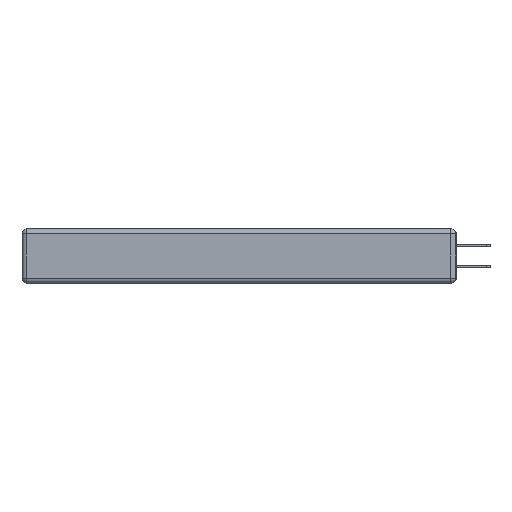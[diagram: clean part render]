
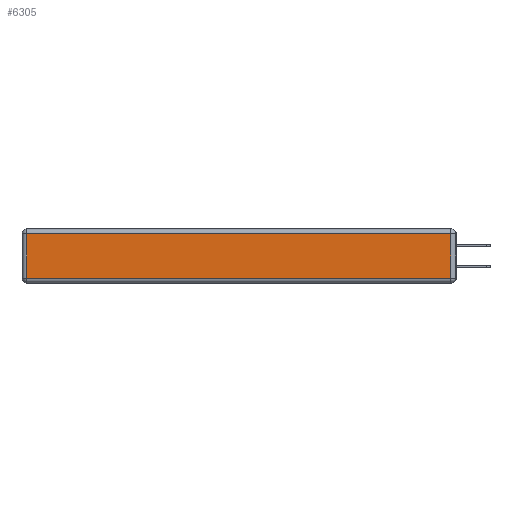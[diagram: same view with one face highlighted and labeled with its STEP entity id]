
A CAD part, left-side view. The second image highlights one B-rep face of the part: STEP entity #6305.
In plain terms, the highlighted planar face has unit normal (-1, 0, 0).
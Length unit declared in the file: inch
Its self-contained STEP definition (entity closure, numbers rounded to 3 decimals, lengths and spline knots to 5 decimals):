
#382 = LINE ( 'NONE', #2606, #5823 ) ;
#821 = ORIENTED_EDGE ( 'NONE', *, *, #4009, .T. ) ;
#872 = LINE ( 'NONE', #3025, #12431 ) ;
#1055 = EDGE_CURVE ( 'NONE', #5582, #9117, #6219, .T. ) ;
#1303 = VERTEX_POINT ( 'NONE', #5323 ) ;
#2340 = CARTESIAN_POINT ( 'NONE',  ( 0., 2.72, -0.313 ) ) ;
#2557 = DIRECTION ( 'NONE',  ( 0., 0., 1. ) ) ;
#2606 = CARTESIAN_POINT ( 'NONE',  ( 0., 0.03, -0.343 ) ) ;
#3025 = CARTESIAN_POINT ( 'NONE',  ( 0., 2.75, -0.03 ) ) ;
#3098 = ORIENTED_EDGE ( 'NONE', *, *, #1055, .T. ) ;
#3707 = AXIS2_PLACEMENT_3D ( 'NONE', #11246, #12403, #5720 ) ;
#3819 = VECTOR ( 'NONE', #5757, 39.37008 ) ;
#4009 = EDGE_CURVE ( 'NONE', #8073, #1303, #872, .T. ) ;
#4342 = CARTESIAN_POINT ( 'NONE',  ( 0., 0.03, -0.313 ) ) ;
#4536 = ORIENTED_EDGE ( 'NONE', *, *, #8718, .T. ) ;
#5294 = EDGE_LOOP ( 'NONE', ( #3098, #4536, #821, #13479 ) ) ;
#5323 = CARTESIAN_POINT ( 'NONE',  ( 0., 2.72, -0.03 ) ) ;
#5582 = VERTEX_POINT ( 'NONE', #2340 ) ;
#5720 = DIRECTION ( 'NONE',  ( 0., 0., 1. ) ) ;
#5757 = DIRECTION ( 'NONE',  ( 0., 0., -1. ) ) ;
#5823 = VECTOR ( 'NONE', #2557, 39.37008 ) ;
#6219 = LINE ( 'NONE', #12802, #9005 ) ;
#6305 = ADVANCED_FACE ( 'NONE', ( #9227 ), #6896, .T. ) ;
#6801 = LINE ( 'NONE', #13356, #3819 ) ;
#6896 = PLANE ( 'NONE',  #3707 ) ;
#7538 = CARTESIAN_POINT ( 'NONE',  ( 0., 0.03, -0.03 ) ) ;
#8073 = VERTEX_POINT ( 'NONE', #7538 ) ;
#8653 = DIRECTION ( 'NONE',  ( 0., 1., 0. ) ) ;
#8718 = EDGE_CURVE ( 'NONE', #9117, #8073, #382, .T. ) ;
#9005 = VECTOR ( 'NONE', #12667, 39.37008 ) ;
#9117 = VERTEX_POINT ( 'NONE', #4342 ) ;
#9227 = FACE_OUTER_BOUND ( 'NONE', #5294, .T. ) ;
#11246 = CARTESIAN_POINT ( 'NONE',  ( 0., 0., -0.343 ) ) ;
#12403 = DIRECTION ( 'NONE',  ( -1., 0., 0. ) ) ;
#12431 = VECTOR ( 'NONE', #8653, 39.37008 ) ;
#12667 = DIRECTION ( 'NONE',  ( 0., -1., 0. ) ) ;
#12802 = CARTESIAN_POINT ( 'NONE',  ( 0., 0., -0.313 ) ) ;
#13165 = EDGE_CURVE ( 'NONE', #1303, #5582, #6801, .T. ) ;
#13356 = CARTESIAN_POINT ( 'NONE',  ( 0., 2.72, -0.343 ) ) ;
#13479 = ORIENTED_EDGE ( 'NONE', *, *, #13165, .T. ) ;
